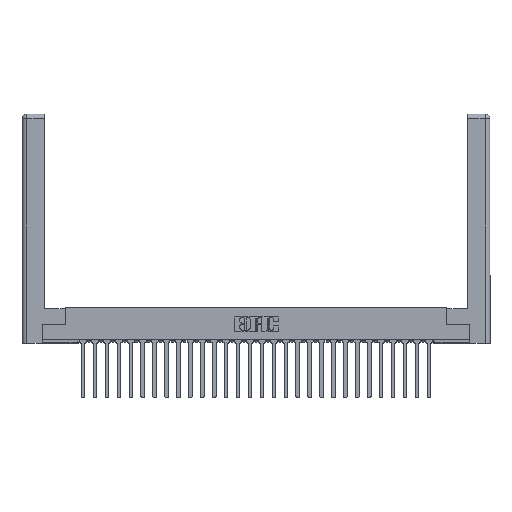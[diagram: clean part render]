
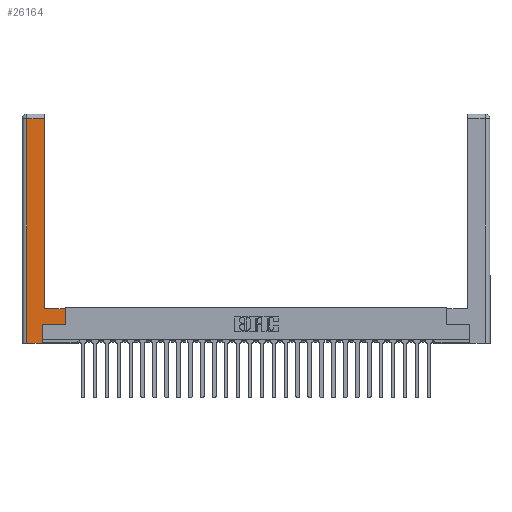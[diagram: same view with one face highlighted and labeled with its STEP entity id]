
A CAD part, top view. The second image highlights one B-rep face of the part: STEP entity #26164.
In plain terms, the highlighted planar face has unit normal (0, 0, 1).
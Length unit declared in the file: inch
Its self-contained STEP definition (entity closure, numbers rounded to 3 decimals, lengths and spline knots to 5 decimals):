
#115 = FACE_OUTER_BOUND ( 'NONE', #9452, .T. ) ;
#358 = VECTOR ( 'NONE', #30484, 39.37008 ) ;
#442 = DIRECTION ( 'NONE',  ( 0., 1., 0. ) ) ;
#520 = VECTOR ( 'NONE', #29651, 39.37008 ) ;
#704 = ORIENTED_EDGE ( 'NONE', *, *, #17051, .T. ) ;
#787 = PLANE ( 'NONE',  #10513 ) ;
#2200 = EDGE_CURVE ( 'NONE', #23149, #29466, #15245, .T. ) ;
#2284 = ORIENTED_EDGE ( 'NONE', *, *, #25629, .T. ) ;
#2464 = CARTESIAN_POINT ( 'NONE',  ( 0.295, 0.45, 0. ) ) ;
#2669 = DIRECTION ( 'NONE',  ( -1., 0., 0. ) ) ;
#3048 = VECTOR ( 'NONE', #13895, 39.37008 ) ;
#3152 = CARTESIAN_POINT ( 'NONE',  ( 0.265, 0.245, 0. ) ) ;
#3861 = EDGE_CURVE ( 'NONE', #29466, #27593, #27762, .T. ) ;
#4159 = ORIENTED_EDGE ( 'NONE', *, *, #19995, .T. ) ;
#4170 = CARTESIAN_POINT ( 'NONE',  ( 0.565, 0.245, 0. ) ) ;
#5115 = ORIENTED_EDGE ( 'NONE', *, *, #22439, .T. ) ;
#5632 = EDGE_CURVE ( 'NONE', #20795, #10821, #15412, .T. ) ;
#5711 = VECTOR ( 'NONE', #7429, 39.37008 ) ;
#6525 = CARTESIAN_POINT ( 'NONE',  ( 0.565, 0.45, 0. ) ) ;
#6567 = ORIENTED_EDGE ( 'NONE', *, *, #2200, .T. ) ;
#6581 = CARTESIAN_POINT ( 'NONE',  ( 0.0615, 0., 0. ) ) ;
#7429 = DIRECTION ( 'NONE',  ( 0., 1., 0. ) ) ;
#7687 = LINE ( 'NONE', #2464, #14026 ) ;
#8300 = ORIENTED_EDGE ( 'NONE', *, *, #3861, .T. ) ;
#8368 = CARTESIAN_POINT ( 'NONE',  ( 0.0615, 2.94, 0. ) ) ;
#8478 = EDGE_CURVE ( 'NONE', #27593, #30413, #17184, .T. ) ;
#9062 = ORIENTED_EDGE ( 'NONE', *, *, #5632, .T. ) ;
#9306 = VERTEX_POINT ( 'NONE', #20113 ) ;
#9452 = EDGE_LOOP ( 'NONE', ( #704, #9062, #5115, #2284, #6567, #8300, #17634, #4159 ) ) ;
#9871 = DIRECTION ( 'NONE',  ( 1., 0., 0. ) ) ;
#10513 = AXIS2_PLACEMENT_3D ( 'NONE', #22690, #15551, #25199 ) ;
#10534 = VERTEX_POINT ( 'NONE', #17582 ) ;
#10821 = VERTEX_POINT ( 'NONE', #22848 ) ;
#10962 = DIRECTION ( 'NONE',  ( 1., 0., 0. ) ) ;
#12400 = CARTESIAN_POINT ( 'NONE',  ( 0.295, 2.94, 0. ) ) ;
#13895 = DIRECTION ( 'NONE',  ( 0., -1., 0. ) ) ;
#14026 = VECTOR ( 'NONE', #2669, 39.37008 ) ;
#14062 = VECTOR ( 'NONE', #9871, 39.37008 ) ;
#15245 = LINE ( 'NONE', #23335, #358 ) ;
#15412 = LINE ( 'NONE', #8368, #520 ) ;
#15551 = DIRECTION ( 'NONE',  ( 0., 0., -1. ) ) ;
#17019 = LINE ( 'NONE', #17337, #14062 ) ;
#17051 = EDGE_CURVE ( 'NONE', #10534, #20795, #20582, .T. ) ;
#17184 = LINE ( 'NONE', #25824, #19729 ) ;
#17337 = CARTESIAN_POINT ( 'NONE',  ( 0.265, 0., 0. ) ) ;
#17582 = CARTESIAN_POINT ( 'NONE',  ( 0.295, 0.45, 0. ) ) ;
#17634 = ORIENTED_EDGE ( 'NONE', *, *, #8478, .T. ) ;
#18672 = LINE ( 'NONE', #6581, #3048 ) ;
#19242 = CARTESIAN_POINT ( 'NONE',  ( 0.265, 0., 0. ) ) ;
#19729 = VECTOR ( 'NONE', #442, 39.37008 ) ;
#19995 = EDGE_CURVE ( 'NONE', #30413, #10534, #7687, .T. ) ;
#20113 = CARTESIAN_POINT ( 'NONE',  ( 0.0615, 0., 0. ) ) ;
#20582 = LINE ( 'NONE', #24051, #5711 ) ;
#20795 = VERTEX_POINT ( 'NONE', #12400 ) ;
#21808 = VECTOR ( 'NONE', #10962, 39.37008 ) ;
#22439 = EDGE_CURVE ( 'NONE', #10821, #9306, #18672, .T. ) ;
#22690 = CARTESIAN_POINT ( 'NONE',  ( 0., 0., 0. ) ) ;
#22848 = CARTESIAN_POINT ( 'NONE',  ( 0.0615, 2.94, 0. ) ) ;
#23149 = VERTEX_POINT ( 'NONE', #19242 ) ;
#23335 = CARTESIAN_POINT ( 'NONE',  ( 0.265, 0.245, 0. ) ) ;
#24051 = CARTESIAN_POINT ( 'NONE',  ( 0.295, 3., 0. ) ) ;
#25199 = DIRECTION ( 'NONE',  ( -1., 0., 0. ) ) ;
#25629 = EDGE_CURVE ( 'NONE', #9306, #23149, #17019, .T. ) ;
#25824 = CARTESIAN_POINT ( 'NONE',  ( 0.565, 0.45, 0. ) ) ;
#26164 = ADVANCED_FACE ( 'NONE', ( #115 ), #787, .F. ) ;
#27593 = VERTEX_POINT ( 'NONE', #30633 ) ;
#27762 = LINE ( 'NONE', #4170, #21808 ) ;
#29466 = VERTEX_POINT ( 'NONE', #3152 ) ;
#29651 = DIRECTION ( 'NONE',  ( -1., 0., 0. ) ) ;
#30413 = VERTEX_POINT ( 'NONE', #6525 ) ;
#30484 = DIRECTION ( 'NONE',  ( 0., 1., 0. ) ) ;
#30633 = CARTESIAN_POINT ( 'NONE',  ( 0.565, 0.245, 0. ) ) ;
